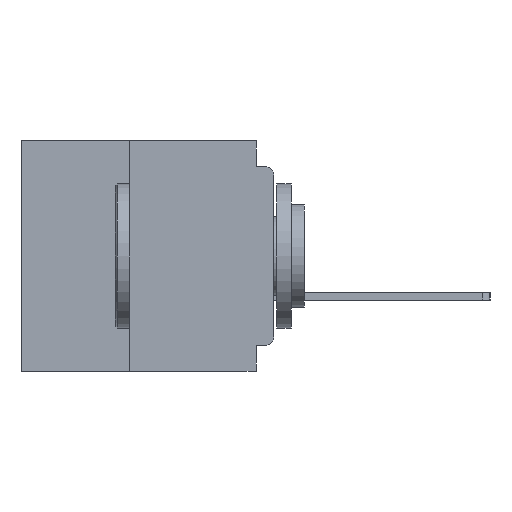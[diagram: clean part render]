
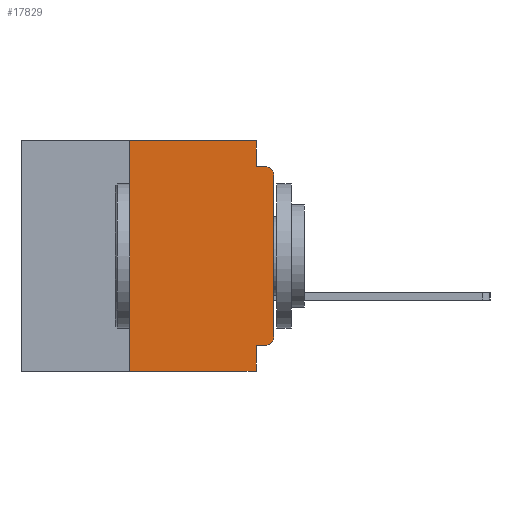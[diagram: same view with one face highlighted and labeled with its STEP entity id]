
A CAD part, left-side view. The second image highlights one B-rep face of the part: STEP entity #17829.
In plain terms, the highlighted planar face has unit normal (-1, 0, 0).
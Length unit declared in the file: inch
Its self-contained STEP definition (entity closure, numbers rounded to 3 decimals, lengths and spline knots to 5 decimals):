
#653 = VECTOR ( 'NONE', #27662, 39.37008 ) ;
#749 = EDGE_CURVE ( 'NONE', #28602, #19115, #51814, .T. ) ;
#816 = AXIS2_PLACEMENT_3D ( 'NONE', #25914, #58031, #30494 ) ;
#883 = CARTESIAN_POINT ( 'NONE',  ( 0., 0.015, -0.045 ) ) ;
#1879 = LINE ( 'NONE', #16681, #37313 ) ;
#2640 = VECTOR ( 'NONE', #46498, 39.37008 ) ;
#5020 = CARTESIAN_POINT ( 'NONE',  ( 0., 0.25, -0.4 ) ) ;
#5329 = CARTESIAN_POINT ( 'NONE',  ( 0., 0.437, 0. ) ) ;
#5978 = CARTESIAN_POINT ( 'NONE',  ( 0., 0.437, 0. ) ) ;
#6649 = EDGE_LOOP ( 'NONE', ( #16383, #47227, #10777, #29387, #15030, #24582, #59370, #40207, #39492, #28474 ) ) ;
#6728 = CARTESIAN_POINT ( 'NONE',  ( 0., 0.015, -0.06 ) ) ;
#8565 = VERTEX_POINT ( 'NONE', #36448 ) ;
#8968 = EDGE_CURVE ( 'NONE', #50515, #44218, #12266, .T. ) ;
#9174 = EDGE_CURVE ( 'NONE', #8565, #44218, #49696, .T. ) ;
#9608 = EDGE_CURVE ( 'NONE', #36209, #8565, #1879, .T. ) ;
#10777 = ORIENTED_EDGE ( 'NONE', *, *, #30906, .F. ) ;
#11464 = DIRECTION ( 'NONE',  ( 0., 0., -1. ) ) ;
#12266 = LINE ( 'NONE', #16558, #47593 ) ;
#12789 = DIRECTION ( 'NONE',  ( 0., 0., -1. ) ) ;
#14508 = FACE_OUTER_BOUND ( 'NONE', #6649, .T. ) ;
#15030 = ORIENTED_EDGE ( 'NONE', *, *, #21927, .F. ) ;
#15597 = CARTESIAN_POINT ( 'NONE',  ( 0., 0.031, 0. ) ) ;
#16383 = ORIENTED_EDGE ( 'NONE', *, *, #48168, .T. ) ;
#16558 = CARTESIAN_POINT ( 'NONE',  ( 0., 0.437, -0.4 ) ) ;
#16681 = CARTESIAN_POINT ( 'NONE',  ( 0., 0., -0.355 ) ) ;
#17829 = ADVANCED_FACE ( 'NONE', ( #14508 ), #42265, .F. ) ;
#18027 = EDGE_CURVE ( 'NONE', #26303, #42123, #53380, .T. ) ;
#19077 = CARTESIAN_POINT ( 'NONE',  ( 0., 0., -0.06 ) ) ;
#19115 = VERTEX_POINT ( 'NONE', #40174 ) ;
#19356 = DIRECTION ( 'NONE',  ( 0., 0., -1. ) ) ;
#20920 = AXIS2_PLACEMENT_3D ( 'NONE', #5329, #46934, #19356 ) ;
#21208 = DIRECTION ( 'NONE',  ( 0., -1., 0. ) ) ;
#21868 = CARTESIAN_POINT ( 'NONE',  ( 0., 0.031, -0.4 ) ) ;
#21927 = EDGE_CURVE ( 'NONE', #39674, #28602, #54284, .T. ) ;
#22429 = CARTESIAN_POINT ( 'NONE',  ( 0., 0., -0.34 ) ) ;
#22787 = CARTESIAN_POINT ( 'NONE',  ( 0., 0.031, -0.4 ) ) ;
#24582 = ORIENTED_EDGE ( 'NONE', *, *, #57046, .F. ) ;
#25914 = CARTESIAN_POINT ( 'NONE',  ( 0., 0.015, -0.34 ) ) ;
#26303 = VERTEX_POINT ( 'NONE', #19077 ) ;
#26598 = EDGE_CURVE ( 'NONE', #36209, #58144, #46562, .T. ) ;
#26732 = VECTOR ( 'NONE', #56231, 39.37008 ) ;
#27662 = DIRECTION ( 'NONE',  ( 0., -1., 0. ) ) ;
#28166 = LINE ( 'NONE', #28514, #26732 ) ;
#28474 = ORIENTED_EDGE ( 'NONE', *, *, #26598, .T. ) ;
#28514 = CARTESIAN_POINT ( 'NONE',  ( 0., 0., 0. ) ) ;
#28602 = VERTEX_POINT ( 'NONE', #57673 ) ;
#28789 = VECTOR ( 'NONE', #12789, 39.37008 ) ;
#29387 = ORIENTED_EDGE ( 'NONE', *, *, #749, .F. ) ;
#30420 = CARTESIAN_POINT ( 'NONE',  ( 0., 0.25, 0. ) ) ;
#30494 = DIRECTION ( 'NONE',  ( 0., 0., -1. ) ) ;
#30906 = EDGE_CURVE ( 'NONE', #19115, #42123, #37588, .T. ) ;
#31789 = DIRECTION ( 'NONE',  ( 0., 0., -1. ) ) ;
#32258 = CARTESIAN_POINT ( 'NONE',  ( 0., 0., -0.045 ) ) ;
#36209 = VERTEX_POINT ( 'NONE', #37854 ) ;
#36448 = CARTESIAN_POINT ( 'NONE',  ( 0., 0.031, -0.355 ) ) ;
#37313 = VECTOR ( 'NONE', #39571, 39.37008 ) ;
#37588 = LINE ( 'NONE', #32258, #653 ) ;
#37854 = CARTESIAN_POINT ( 'NONE',  ( 0., 0.015, -0.355 ) ) ;
#38838 = VECTOR ( 'NONE', #31789, 39.37008 ) ;
#38986 = DIRECTION ( 'NONE',  ( -1., 0., 0. ) ) ;
#39492 = ORIENTED_EDGE ( 'NONE', *, *, #9608, .F. ) ;
#39529 = LINE ( 'NONE', #55498, #2640 ) ;
#39571 = DIRECTION ( 'NONE',  ( 0., 1., 0. ) ) ;
#39674 = VERTEX_POINT ( 'NONE', #30420 ) ;
#40174 = CARTESIAN_POINT ( 'NONE',  ( 0., 0.031, -0.045 ) ) ;
#40207 = ORIENTED_EDGE ( 'NONE', *, *, #9174, .F. ) ;
#42047 = VECTOR ( 'NONE', #47603, 39.37008 ) ;
#42123 = VERTEX_POINT ( 'NONE', #883 ) ;
#42265 = PLANE ( 'NONE',  #20920 ) ;
#44218 = VERTEX_POINT ( 'NONE', #21868 ) ;
#46498 = DIRECTION ( 'NONE',  ( 0., 0., 1. ) ) ;
#46562 = CIRCLE ( 'NONE', #816, 0.015 ) ;
#46934 = DIRECTION ( 'NONE',  ( 1., 0., 0. ) ) ;
#47227 = ORIENTED_EDGE ( 'NONE', *, *, #18027, .T. ) ;
#47593 = VECTOR ( 'NONE', #21208, 39.37008 ) ;
#47603 = DIRECTION ( 'NONE',  ( 0., -1., 0. ) ) ;
#48168 = EDGE_CURVE ( 'NONE', #58144, #26303, #28166, .T. ) ;
#49696 = LINE ( 'NONE', #22787, #38838 ) ;
#50515 = VERTEX_POINT ( 'NONE', #5020 ) ;
#51814 = LINE ( 'NONE', #15597, #28789 ) ;
#53380 = CIRCLE ( 'NONE', #54798, 0.015 ) ;
#54284 = LINE ( 'NONE', #5978, #42047 ) ;
#54798 = AXIS2_PLACEMENT_3D ( 'NONE', #6728, #38986, #11464 ) ;
#55498 = CARTESIAN_POINT ( 'NONE',  ( 0., 0.25, -0.4 ) ) ;
#56231 = DIRECTION ( 'NONE',  ( 0., 0., 1. ) ) ;
#57046 = EDGE_CURVE ( 'NONE', #50515, #39674, #39529, .T. ) ;
#57673 = CARTESIAN_POINT ( 'NONE',  ( 0., 0.031, 0. ) ) ;
#58031 = DIRECTION ( 'NONE',  ( -1., 0., 0. ) ) ;
#58144 = VERTEX_POINT ( 'NONE', #22429 ) ;
#59370 = ORIENTED_EDGE ( 'NONE', *, *, #8968, .T. ) ;
